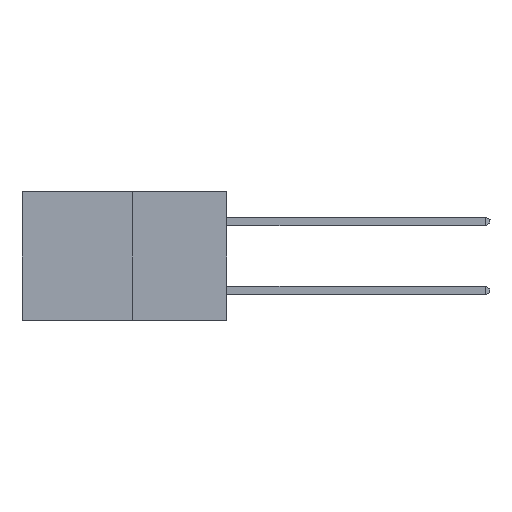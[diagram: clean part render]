
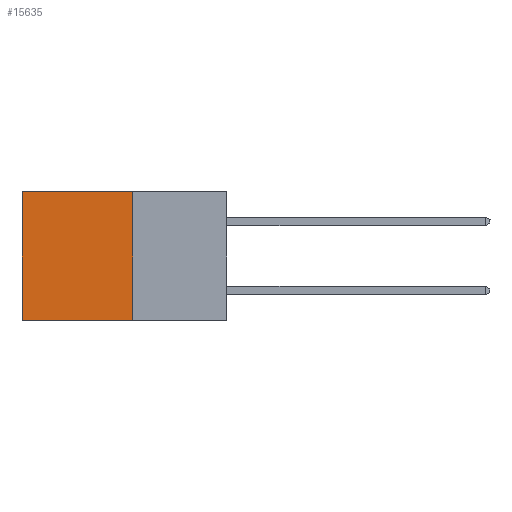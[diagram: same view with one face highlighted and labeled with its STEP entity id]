
A CAD part, left-side view. The second image highlights one B-rep face of the part: STEP entity #15635.
In plain terms, the highlighted planar face has unit normal (-1, 0, 0).
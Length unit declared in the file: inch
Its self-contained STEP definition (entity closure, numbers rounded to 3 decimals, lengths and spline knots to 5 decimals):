
#1571 = ORIENTED_EDGE ( 'NONE', *, *, #10547, .T. ) ;
#1652 = DIRECTION ( 'NONE',  ( 1., 0., 0. ) ) ;
#2153 = DIRECTION ( 'NONE',  ( 0., 1., 0. ) ) ;
#2291 = LINE ( 'NONE', #19399, #11898 ) ;
#3034 = VERTEX_POINT ( 'NONE', #15404 ) ;
#3807 = VECTOR ( 'NONE', #23120, 39.37008 ) ;
#5383 = VECTOR ( 'NONE', #6813, 39.37008 ) ;
#5478 = EDGE_CURVE ( 'NONE', #6918, #20220, #5958, .T. ) ;
#5958 = LINE ( 'NONE', #21149, #5383 ) ;
#6708 = ORIENTED_EDGE ( 'NONE', *, *, #18668, .F. ) ;
#6813 = DIRECTION ( 'NONE',  ( 0., 0., -1. ) ) ;
#6918 = VERTEX_POINT ( 'NONE', #21564 ) ;
#7562 = VECTOR ( 'NONE', #2153, 39.37008 ) ;
#8983 = CARTESIAN_POINT ( 'NONE',  ( 0.277, 0.59, 0. ) ) ;
#9966 = FACE_OUTER_BOUND ( 'NONE', #18529, .T. ) ;
#10547 = EDGE_CURVE ( 'NONE', #6918, #12091, #13400, .T. ) ;
#11802 = ORIENTED_EDGE ( 'NONE', *, *, #5478, .F. ) ;
#11898 = VECTOR ( 'NONE', #21210, 39.37008 ) ;
#12091 = VERTEX_POINT ( 'NONE', #8983 ) ;
#12654 = EDGE_CURVE ( 'NONE', #12091, #3034, #2291, .T. ) ;
#13400 = LINE ( 'NONE', #21318, #3807 ) ;
#13604 = CARTESIAN_POINT ( 'NONE',  ( 0.277, 0.27, -0.37 ) ) ;
#14267 = DIRECTION ( 'NONE',  ( 0., 0., -1. ) ) ;
#14758 = CARTESIAN_POINT ( 'NONE',  ( 0.277, 0.27, -0.37 ) ) ;
#15404 = CARTESIAN_POINT ( 'NONE',  ( 0.277, 0.59, -0.37 ) ) ;
#15635 = ADVANCED_FACE ( 'NONE', ( #9966 ), #21381, .F. ) ;
#16376 = AXIS2_PLACEMENT_3D ( 'NONE', #23174, #1652, #14267 ) ;
#17046 = LINE ( 'NONE', #14758, #7562 ) ;
#18529 = EDGE_LOOP ( 'NONE', ( #21417, #6708, #11802, #1571 ) ) ;
#18668 = EDGE_CURVE ( 'NONE', #20220, #3034, #17046, .T. ) ;
#19399 = CARTESIAN_POINT ( 'NONE',  ( 0.277, 0.59, -0.37 ) ) ;
#20220 = VERTEX_POINT ( 'NONE', #13604 ) ;
#21149 = CARTESIAN_POINT ( 'NONE',  ( 0.277, 0.27, -0.37 ) ) ;
#21210 = DIRECTION ( 'NONE',  ( 0., 0., -1. ) ) ;
#21318 = CARTESIAN_POINT ( 'NONE',  ( 0.277, 0.27, 0. ) ) ;
#21381 = PLANE ( 'NONE',  #16376 ) ;
#21417 = ORIENTED_EDGE ( 'NONE', *, *, #12654, .T. ) ;
#21564 = CARTESIAN_POINT ( 'NONE',  ( 0.277, 0.27, 0. ) ) ;
#23120 = DIRECTION ( 'NONE',  ( 0., 1., 0. ) ) ;
#23174 = CARTESIAN_POINT ( 'NONE',  ( 0.277, 0.27, -0.37 ) ) ;
